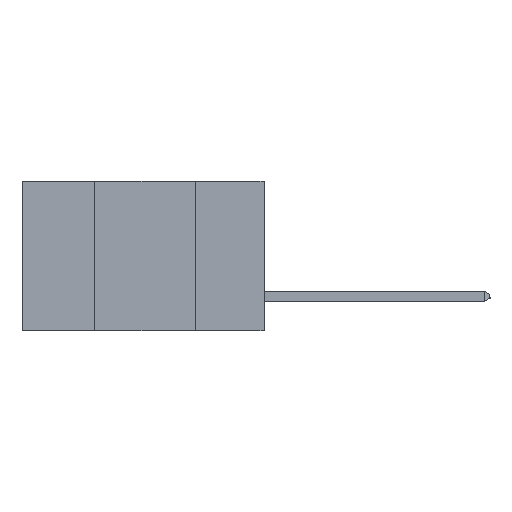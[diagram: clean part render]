
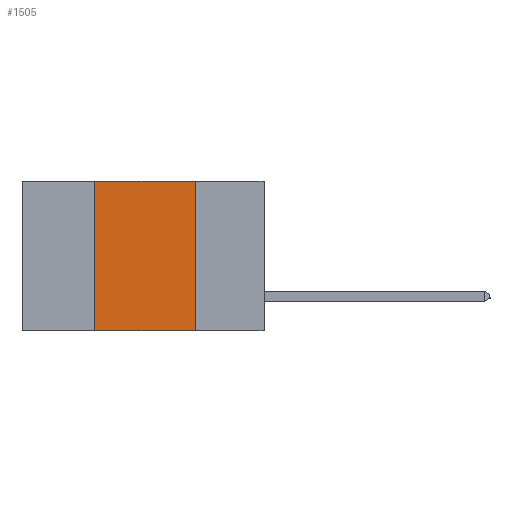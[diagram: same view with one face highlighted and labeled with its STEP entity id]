
A CAD part, left-side view. The second image highlights one B-rep face of the part: STEP entity #1505.
In plain terms, the highlighted planar face has unit normal (-1, 0, 0).
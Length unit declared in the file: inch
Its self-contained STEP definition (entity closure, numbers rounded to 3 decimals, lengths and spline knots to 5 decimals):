
#69 = CARTESIAN_POINT ( 'NONE',  ( 0., 0.6, -0.37 ) ) ;
#739 = LINE ( 'NONE', #4082, #2584 ) ;
#889 = CARTESIAN_POINT ( 'NONE',  ( 0., 0.42, -0.37 ) ) ;
#1176 = AXIS2_PLACEMENT_3D ( 'NONE', #3385, #10598, #7673 ) ;
#1505 = ADVANCED_FACE ( 'NONE', ( #7271 ), #10594, .F. ) ;
#2083 = LINE ( 'NONE', #9679, #6441 ) ;
#2092 = VECTOR ( 'NONE', #6489, 39.37008 ) ;
#2198 = VERTEX_POINT ( 'NONE', #6015 ) ;
#2380 = EDGE_CURVE ( 'NONE', #5027, #6711, #2083, .T. ) ;
#2458 = ORIENTED_EDGE ( 'NONE', *, *, #6662, .F. ) ;
#2584 = VECTOR ( 'NONE', #9954, 39.37008 ) ;
#3064 = CARTESIAN_POINT ( 'NONE',  ( 0., 0.6, 0. ) ) ;
#3199 = CARTESIAN_POINT ( 'NONE',  ( 0., 0.17, -0.37 ) ) ;
#3385 = CARTESIAN_POINT ( 'NONE',  ( 0., 0.6, 0. ) ) ;
#3876 = EDGE_LOOP ( 'NONE', ( #5337, #9806, #2458, #9292 ) ) ;
#4082 = CARTESIAN_POINT ( 'NONE',  ( 0., 0.42, 0. ) ) ;
#4932 = CARTESIAN_POINT ( 'NONE',  ( 0., 0.17, 0. ) ) ;
#5027 = VERTEX_POINT ( 'NONE', #4932 ) ;
#5337 = ORIENTED_EDGE ( 'NONE', *, *, #2380, .F. ) ;
#6015 = CARTESIAN_POINT ( 'NONE',  ( 0., 0.42, 0. ) ) ;
#6097 = EDGE_CURVE ( 'NONE', #8203, #6711, #10407, .T. ) ;
#6441 = VECTOR ( 'NONE', #9804, 39.37008 ) ;
#6489 = DIRECTION ( 'NONE',  ( 0., -1., 0. ) ) ;
#6662 = EDGE_CURVE ( 'NONE', #8203, #2198, #739, .T. ) ;
#6711 = VERTEX_POINT ( 'NONE', #3199 ) ;
#6980 = LINE ( 'NONE', #3064, #2092 ) ;
#7271 = FACE_OUTER_BOUND ( 'NONE', #3876, .T. ) ;
#7673 = DIRECTION ( 'NONE',  ( 0., 0., -1. ) ) ;
#8203 = VERTEX_POINT ( 'NONE', #889 ) ;
#9292 = ORIENTED_EDGE ( 'NONE', *, *, #6097, .T. ) ;
#9337 = EDGE_CURVE ( 'NONE', #2198, #5027, #6980, .T. ) ;
#9679 = CARTESIAN_POINT ( 'NONE',  ( 0., 0.17, 0. ) ) ;
#9804 = DIRECTION ( 'NONE',  ( 0., 0., -1. ) ) ;
#9806 = ORIENTED_EDGE ( 'NONE', *, *, #9337, .F. ) ;
#9954 = DIRECTION ( 'NONE',  ( 0., 0., 1. ) ) ;
#10166 = VECTOR ( 'NONE', #10405, 39.37008 ) ;
#10405 = DIRECTION ( 'NONE',  ( 0., -1., 0. ) ) ;
#10407 = LINE ( 'NONE', #69, #10166 ) ;
#10594 = PLANE ( 'NONE',  #1176 ) ;
#10598 = DIRECTION ( 'NONE',  ( 1., 0., 0. ) ) ;
